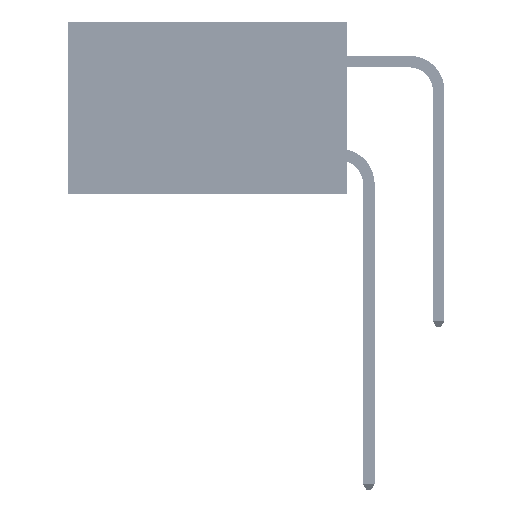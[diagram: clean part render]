
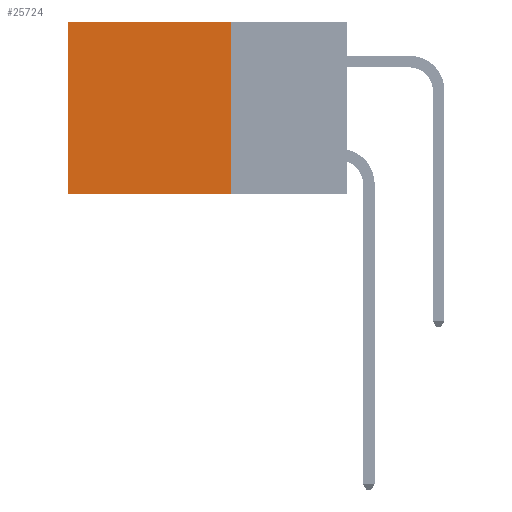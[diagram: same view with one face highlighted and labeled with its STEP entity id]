
A CAD part, left-side view. The second image highlights one B-rep face of the part: STEP entity #25724.
In plain terms, the highlighted planar face has unit normal (-1, 0, 0).
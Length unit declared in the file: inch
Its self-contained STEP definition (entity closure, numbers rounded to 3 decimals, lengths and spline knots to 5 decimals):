
#2552 = VECTOR ( 'NONE', #4979, 39.37008 ) ;
#4699 = CARTESIAN_POINT ( 'NONE',  ( 0.2875, 0.6, -0.37 ) ) ;
#4979 = DIRECTION ( 'NONE',  ( 0., 0., -1. ) ) ;
#8332 = VERTEX_POINT ( 'NONE', #38235 ) ;
#9445 = LINE ( 'NONE', #17560, #18607 ) ;
#9870 = DIRECTION ( 'NONE',  ( 0., 0., -1. ) ) ;
#10911 = DIRECTION ( 'NONE',  ( 0., 1., 0. ) ) ;
#12201 = AXIS2_PLACEMENT_3D ( 'NONE', #40561, #40043, #48486 ) ;
#12618 = LINE ( 'NONE', #39205, #13845 ) ;
#13845 = VECTOR ( 'NONE', #27300, 39.37008 ) ;
#14017 = VERTEX_POINT ( 'NONE', #4699 ) ;
#16365 = ORIENTED_EDGE ( 'NONE', *, *, #40967, .F. ) ;
#16614 = CARTESIAN_POINT ( 'NONE',  ( 0.2875, 0.6, 0. ) ) ;
#17560 = CARTESIAN_POINT ( 'NONE',  ( 0.2875, 0.25, 0. ) ) ;
#18607 = VECTOR ( 'NONE', #9870, 39.37008 ) ;
#20877 = EDGE_LOOP ( 'NONE', ( #39689, #43663, #16365, #24685 ) ) ;
#21585 = VERTEX_POINT ( 'NONE', #24693 ) ;
#23346 = LINE ( 'NONE', #16614, #2552 ) ;
#24685 = ORIENTED_EDGE ( 'NONE', *, *, #31370, .T. ) ;
#24693 = CARTESIAN_POINT ( 'NONE',  ( 0.2875, 0.25, -0.37 ) ) ;
#25724 = ADVANCED_FACE ( 'NONE', ( #48035 ), #36610, .F. ) ;
#27300 = DIRECTION ( 'NONE',  ( 0., 1., 0. ) ) ;
#30393 = CARTESIAN_POINT ( 'NONE',  ( 0.2875, 0.25, -0.37 ) ) ;
#31370 = EDGE_CURVE ( 'NONE', #8332, #39429, #12618, .T. ) ;
#32404 = CARTESIAN_POINT ( 'NONE',  ( 0.2875, 0.6, 0. ) ) ;
#35371 = EDGE_CURVE ( 'NONE', #39429, #14017, #23346, .T. ) ;
#36377 = LINE ( 'NONE', #30393, #48676 ) ;
#36610 = PLANE ( 'NONE',  #12201 ) ;
#38235 = CARTESIAN_POINT ( 'NONE',  ( 0.2875, 0.25, 0. ) ) ;
#39205 = CARTESIAN_POINT ( 'NONE',  ( 0.2875, 0.25, 0. ) ) ;
#39429 = VERTEX_POINT ( 'NONE', #32404 ) ;
#39689 = ORIENTED_EDGE ( 'NONE', *, *, #35371, .T. ) ;
#40043 = DIRECTION ( 'NONE',  ( 1., 0., 0. ) ) ;
#40561 = CARTESIAN_POINT ( 'NONE',  ( 0.2875, 0.25, 0. ) ) ;
#40967 = EDGE_CURVE ( 'NONE', #8332, #21585, #9445, .T. ) ;
#41241 = EDGE_CURVE ( 'NONE', #21585, #14017, #36377, .T. ) ;
#43663 = ORIENTED_EDGE ( 'NONE', *, *, #41241, .F. ) ;
#48035 = FACE_OUTER_BOUND ( 'NONE', #20877, .T. ) ;
#48486 = DIRECTION ( 'NONE',  ( 0., 0., -1. ) ) ;
#48676 = VECTOR ( 'NONE', #10911, 39.37008 ) ;
